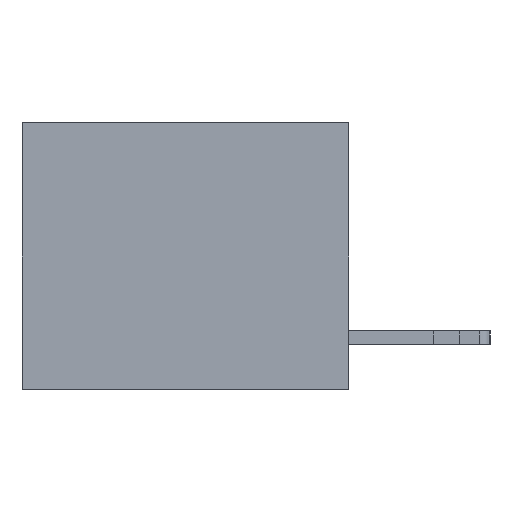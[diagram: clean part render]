
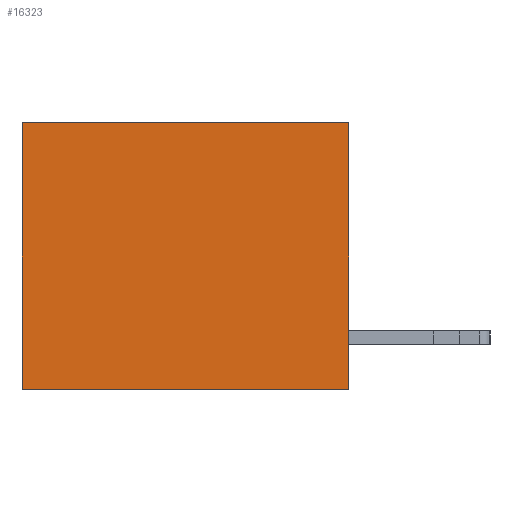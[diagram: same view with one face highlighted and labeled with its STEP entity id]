
A CAD part, left-side view. The second image highlights one B-rep face of the part: STEP entity #16323.
In plain terms, the highlighted planar face has unit normal (-1, 0, 0).
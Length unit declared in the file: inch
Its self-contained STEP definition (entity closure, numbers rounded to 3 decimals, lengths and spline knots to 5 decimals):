
#222 = ORIENTED_EDGE ( 'NONE', *, *, #5377, .F. ) ;
#1192 = EDGE_LOOP ( 'NONE', ( #8535, #8600, #222, #18171 ) ) ;
#2059 = AXIS2_PLACEMENT_3D ( 'NONE', #12139, #16564, #15249 ) ;
#2962 = CARTESIAN_POINT ( 'NONE',  ( 0.3165, 0.6, -0.49 ) ) ;
#3208 = DIRECTION ( 'NONE',  ( 0., 1., 0. ) ) ;
#3641 = VECTOR ( 'NONE', #3208, 39.37008 ) ;
#3677 = VERTEX_POINT ( 'NONE', #2962 ) ;
#4924 = CARTESIAN_POINT ( 'NONE',  ( 0.3165, 0.6, -0.49 ) ) ;
#5221 = EDGE_CURVE ( 'NONE', #15555, #14912, #12604, .T. ) ;
#5377 = EDGE_CURVE ( 'NONE', #15555, #16449, #17818, .T. ) ;
#6449 = EDGE_CURVE ( 'NONE', #16449, #3677, #10819, .T. ) ;
#7832 = CARTESIAN_POINT ( 'NONE',  ( 0.3165, 0., 0. ) ) ;
#7891 = VECTOR ( 'NONE', #16043, 39.37008 ) ;
#8535 = ORIENTED_EDGE ( 'NONE', *, *, #14753, .T. ) ;
#8600 = ORIENTED_EDGE ( 'NONE', *, *, #6449, .F. ) ;
#8749 = PLANE ( 'NONE',  #2059 ) ;
#10084 = FACE_OUTER_BOUND ( 'NONE', #1192, .T. ) ;
#10292 = DIRECTION ( 'NONE',  ( 0., 1., 0. ) ) ;
#10819 = LINE ( 'NONE', #13485, #16264 ) ;
#11452 = CARTESIAN_POINT ( 'NONE',  ( 0.3165, 0., 0. ) ) ;
#12139 = CARTESIAN_POINT ( 'NONE',  ( 0.3165, 0., -0.49 ) ) ;
#12604 = LINE ( 'NONE', #11452, #3641 ) ;
#13485 = CARTESIAN_POINT ( 'NONE',  ( 0.3165, 0., -0.49 ) ) ;
#14721 = CARTESIAN_POINT ( 'NONE',  ( 0.3165, 0.6, 0. ) ) ;
#14753 = EDGE_CURVE ( 'NONE', #14912, #3677, #17020, .T. ) ;
#14912 = VERTEX_POINT ( 'NONE', #14721 ) ;
#14916 = CARTESIAN_POINT ( 'NONE',  ( 0.3165, 0., -0.49 ) ) ;
#15249 = DIRECTION ( 'NONE',  ( 0., 0., -1. ) ) ;
#15555 = VERTEX_POINT ( 'NONE', #7832 ) ;
#15998 = CARTESIAN_POINT ( 'NONE',  ( 0.3165, 0., -0.49 ) ) ;
#16043 = DIRECTION ( 'NONE',  ( 0., 0., -1. ) ) ;
#16264 = VECTOR ( 'NONE', #10292, 39.37008 ) ;
#16323 = ADVANCED_FACE ( 'NONE', ( #10084 ), #8749, .F. ) ;
#16449 = VERTEX_POINT ( 'NONE', #15998 ) ;
#16564 = DIRECTION ( 'NONE',  ( 1., 0., 0. ) ) ;
#17020 = LINE ( 'NONE', #4924, #7891 ) ;
#17818 = LINE ( 'NONE', #14916, #18816 ) ;
#18171 = ORIENTED_EDGE ( 'NONE', *, *, #5221, .T. ) ;
#18816 = VECTOR ( 'NONE', #19716, 39.37008 ) ;
#19716 = DIRECTION ( 'NONE',  ( 0., 0., -1. ) ) ;
